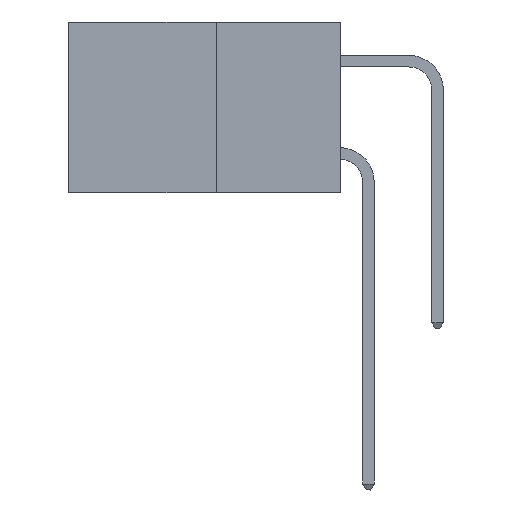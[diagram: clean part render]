
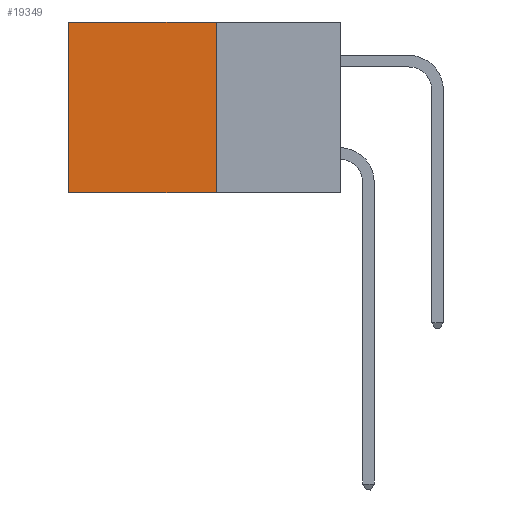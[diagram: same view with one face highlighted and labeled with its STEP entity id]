
A CAD part, left-side view. The second image highlights one B-rep face of the part: STEP entity #19349.
In plain terms, the highlighted planar face has unit normal (-1, 0, 0).
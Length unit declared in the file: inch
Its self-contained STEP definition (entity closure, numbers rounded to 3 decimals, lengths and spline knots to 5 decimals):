
#330 = ORIENTED_EDGE ( 'NONE', *, *, #8921, .F. ) ;
#424 = LINE ( 'NONE', #3638, #17215 ) ;
#609 = LINE ( 'NONE', #5248, #9768 ) ;
#1378 = DIRECTION ( 'NONE',  ( 0., 1., 0. ) ) ;
#1605 = CARTESIAN_POINT ( 'NONE',  ( 0.277, 0.27, 0. ) ) ;
#2235 = VERTEX_POINT ( 'NONE', #4397 ) ;
#2257 = CARTESIAN_POINT ( 'NONE',  ( 0.277, 0.27, -0.37 ) ) ;
#3638 = CARTESIAN_POINT ( 'NONE',  ( 0.277, 0.27, -0.37 ) ) ;
#3709 = DIRECTION ( 'NONE',  ( 0., 0., -1. ) ) ;
#4046 = EDGE_LOOP ( 'NONE', ( #20878, #8508, #330, #4715 ) ) ;
#4115 = EDGE_CURVE ( 'NONE', #8146, #2235, #609, .T. ) ;
#4397 = CARTESIAN_POINT ( 'NONE',  ( 0.277, 0.59, -0.37 ) ) ;
#4715 = ORIENTED_EDGE ( 'NONE', *, *, #8797, .T. ) ;
#4879 = VERTEX_POINT ( 'NONE', #20843 ) ;
#5248 = CARTESIAN_POINT ( 'NONE',  ( 0.277, 0.59, -0.37 ) ) ;
#5297 = DIRECTION ( 'NONE',  ( 0., 0., -1. ) ) ;
#7565 = DIRECTION ( 'NONE',  ( 0., 0., -1. ) ) ;
#8146 = VERTEX_POINT ( 'NONE', #13330 ) ;
#8200 = EDGE_CURVE ( 'NONE', #9702, #2235, #14250, .T. ) ;
#8508 = ORIENTED_EDGE ( 'NONE', *, *, #8200, .F. ) ;
#8797 = EDGE_CURVE ( 'NONE', #4879, #8146, #15998, .T. ) ;
#8921 = EDGE_CURVE ( 'NONE', #4879, #9702, #424, .T. ) ;
#9376 = VECTOR ( 'NONE', #11998, 39.37008 ) ;
#9702 = VERTEX_POINT ( 'NONE', #2257 ) ;
#9768 = VECTOR ( 'NONE', #3709, 39.37008 ) ;
#11148 = VECTOR ( 'NONE', #1378, 39.37008 ) ;
#11707 = FACE_OUTER_BOUND ( 'NONE', #4046, .T. ) ;
#11998 = DIRECTION ( 'NONE',  ( 0., 1., 0. ) ) ;
#12074 = CARTESIAN_POINT ( 'NONE',  ( 0.277, 0.27, -0.37 ) ) ;
#13330 = CARTESIAN_POINT ( 'NONE',  ( 0.277, 0.59, 0. ) ) ;
#14039 = PLANE ( 'NONE',  #15087 ) ;
#14250 = LINE ( 'NONE', #12074, #9376 ) ;
#15087 = AXIS2_PLACEMENT_3D ( 'NONE', #15684, #17269, #7565 ) ;
#15684 = CARTESIAN_POINT ( 'NONE',  ( 0.277, 0.27, -0.37 ) ) ;
#15998 = LINE ( 'NONE', #1605, #11148 ) ;
#17215 = VECTOR ( 'NONE', #5297, 39.37008 ) ;
#17269 = DIRECTION ( 'NONE',  ( 1., 0., 0. ) ) ;
#19349 = ADVANCED_FACE ( 'NONE', ( #11707 ), #14039, .F. ) ;
#20843 = CARTESIAN_POINT ( 'NONE',  ( 0.277, 0.27, 0. ) ) ;
#20878 = ORIENTED_EDGE ( 'NONE', *, *, #4115, .T. ) ;
